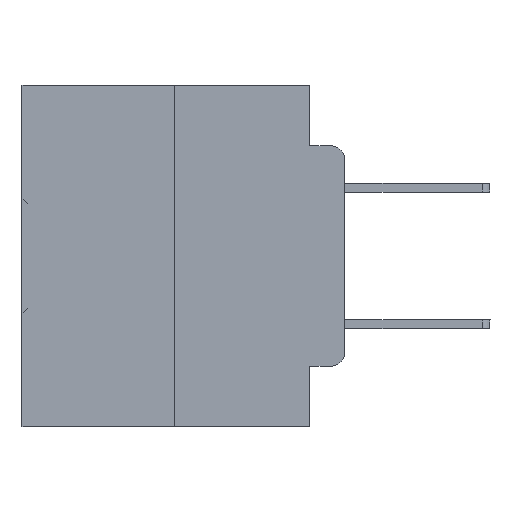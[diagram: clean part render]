
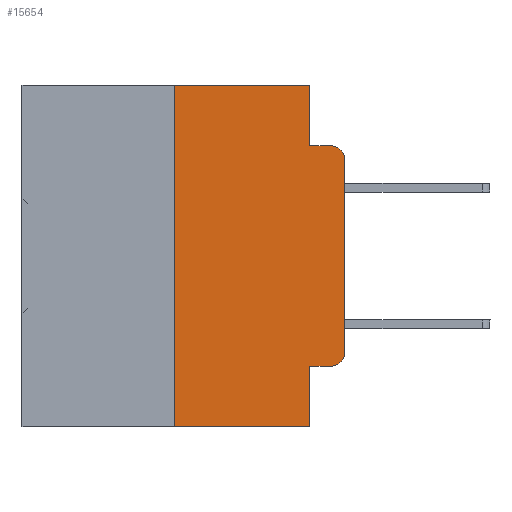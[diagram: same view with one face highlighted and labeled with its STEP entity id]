
A CAD part, left-side view. The second image highlights one B-rep face of the part: STEP entity #15654.
In plain terms, the highlighted planar face has unit normal (-1, 0, 0).
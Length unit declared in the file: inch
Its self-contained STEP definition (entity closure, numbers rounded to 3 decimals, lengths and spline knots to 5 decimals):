
#1027 = LINE ( 'NONE', #9541, #3161 ) ;
#1177 = CARTESIAN_POINT ( 'NONE',  ( 0., 0.051, 0. ) ) ;
#1514 = VERTEX_POINT ( 'NONE', #17725 ) ;
#2188 = CARTESIAN_POINT ( 'NONE',  ( 0., 0.051, -0.5 ) ) ;
#2288 = DIRECTION ( 'NONE',  ( 0., 0., -1. ) ) ;
#2424 = VECTOR ( 'NONE', #8841, 39.37008 ) ;
#2534 = CARTESIAN_POINT ( 'NONE',  ( 0., 0.051, 0. ) ) ;
#3006 = ORIENTED_EDGE ( 'NONE', *, *, #20452, .T. ) ;
#3094 = EDGE_CURVE ( 'NONE', #30216, #5274, #14071, .T. ) ;
#3161 = VECTOR ( 'NONE', #12062, 39.37008 ) ;
#3354 = CARTESIAN_POINT ( 'NONE',  ( 0., 0.25, -0.5 ) ) ;
#3765 = EDGE_CURVE ( 'NONE', #20143, #28749, #12743, .T. ) ;
#3801 = EDGE_CURVE ( 'NONE', #28749, #17695, #10401, .T. ) ;
#3813 = CARTESIAN_POINT ( 'NONE',  ( 0., 0.02, -0.4115 ) ) ;
#4164 = LINE ( 'NONE', #6699, #22034 ) ;
#4438 = DIRECTION ( 'NONE',  ( 0., 0., 1. ) ) ;
#4473 = AXIS2_PLACEMENT_3D ( 'NONE', #16022, #18914, #2288 ) ;
#4555 = VERTEX_POINT ( 'NONE', #6662 ) ;
#5274 = VERTEX_POINT ( 'NONE', #24981 ) ;
#5427 = VERTEX_POINT ( 'NONE', #3813 ) ;
#5631 = AXIS2_PLACEMENT_3D ( 'NONE', #7653, #18507, #7835 ) ;
#5682 = AXIS2_PLACEMENT_3D ( 'NONE', #30928, #16939, #17121 ) ;
#6244 = EDGE_CURVE ( 'NONE', #20143, #10310, #13314, .T. ) ;
#6662 = CARTESIAN_POINT ( 'NONE',  ( 0., 0., -0.3915 ) ) ;
#6699 = CARTESIAN_POINT ( 'NONE',  ( 0., 0.051, -0.4115 ) ) ;
#7653 = CARTESIAN_POINT ( 'NONE',  ( 0., 0.02, -0.3915 ) ) ;
#7835 = DIRECTION ( 'NONE',  ( 0., 0., -1. ) ) ;
#8578 = VECTOR ( 'NONE', #4438, 39.37008 ) ;
#8841 = DIRECTION ( 'NONE',  ( 0., -1., 0. ) ) ;
#9029 = ORIENTED_EDGE ( 'NONE', *, *, #3765, .F. ) ;
#9263 = ORIENTED_EDGE ( 'NONE', *, *, #3801, .F. ) ;
#9541 = CARTESIAN_POINT ( 'NONE',  ( 0., 0., 0. ) ) ;
#9544 = PLANE ( 'NONE',  #4473 ) ;
#10310 = VERTEX_POINT ( 'NONE', #2188 ) ;
#10401 = LINE ( 'NONE', #15629, #20732 ) ;
#10429 = EDGE_CURVE ( 'NONE', #17695, #30216, #16269, .T. ) ;
#11016 = DIRECTION ( 'NONE',  ( 0., 0., -1. ) ) ;
#11027 = EDGE_LOOP ( 'NONE', ( #29076, #34854, #33288, #33503, #9263, #9029, #14259, #21381, #15442, #3006 ) ) ;
#11551 = CARTESIAN_POINT ( 'NONE',  ( 0., 0.051, -0.0885 ) ) ;
#12062 = DIRECTION ( 'NONE',  ( 0., 0., 1. ) ) ;
#12265 = VECTOR ( 'NONE', #11016, 39.37008 ) ;
#12601 = EDGE_CURVE ( 'NONE', #4555, #27431, #1027, .T. ) ;
#12743 = LINE ( 'NONE', #26514, #8578 ) ;
#13314 = LINE ( 'NONE', #21302, #19636 ) ;
#14071 = LINE ( 'NONE', #11551, #2424 ) ;
#14259 = ORIENTED_EDGE ( 'NONE', *, *, #6244, .T. ) ;
#15009 = CARTESIAN_POINT ( 'NONE',  ( 0., 0.051, 0. ) ) ;
#15442 = ORIENTED_EDGE ( 'NONE', *, *, #30143, .T. ) ;
#15629 = CARTESIAN_POINT ( 'NONE',  ( 0., 0.473, 0. ) ) ;
#15654 = ADVANCED_FACE ( 'NONE', ( #34362 ), #9544, .F. ) ;
#16022 = CARTESIAN_POINT ( 'NONE',  ( 0., 0.473, 0. ) ) ;
#16269 = LINE ( 'NONE', #2534, #12265 ) ;
#16939 = DIRECTION ( 'NONE',  ( -1., 0., 0. ) ) ;
#17121 = DIRECTION ( 'NONE',  ( 0., 0., -1. ) ) ;
#17695 = VERTEX_POINT ( 'NONE', #15009 ) ;
#17725 = CARTESIAN_POINT ( 'NONE',  ( 0., 0.051, -0.4115 ) ) ;
#18507 = DIRECTION ( 'NONE',  ( -1., 0., 0. ) ) ;
#18718 = DIRECTION ( 'NONE',  ( 0., -1., 0. ) ) ;
#18914 = DIRECTION ( 'NONE',  ( 1., 0., 0. ) ) ;
#19356 = CARTESIAN_POINT ( 'NONE',  ( 0., 0.25, 0. ) ) ;
#19636 = VECTOR ( 'NONE', #21655, 39.37008 ) ;
#20143 = VERTEX_POINT ( 'NONE', #3354 ) ;
#20157 = CIRCLE ( 'NONE', #5682, 0.02 ) ;
#20447 = CARTESIAN_POINT ( 'NONE',  ( 0., 0.051, -0.0885 ) ) ;
#20452 = EDGE_CURVE ( 'NONE', #5427, #4555, #34583, .T. ) ;
#20732 = VECTOR ( 'NONE', #18718, 39.37008 ) ;
#21302 = CARTESIAN_POINT ( 'NONE',  ( 0., 0.473, -0.5 ) ) ;
#21381 = ORIENTED_EDGE ( 'NONE', *, *, #21713, .F. ) ;
#21576 = EDGE_CURVE ( 'NONE', #27431, #5274, #20157, .T. ) ;
#21655 = DIRECTION ( 'NONE',  ( 0., -1., 0. ) ) ;
#21713 = EDGE_CURVE ( 'NONE', #1514, #10310, #34508, .T. ) ;
#22034 = VECTOR ( 'NONE', #23704, 39.37008 ) ;
#22763 = CARTESIAN_POINT ( 'NONE',  ( 0., 0., -0.1085 ) ) ;
#23459 = DIRECTION ( 'NONE',  ( 0., 0., -1. ) ) ;
#23704 = DIRECTION ( 'NONE',  ( 0., -1., 0. ) ) ;
#24981 = CARTESIAN_POINT ( 'NONE',  ( 0., 0.02, -0.0885 ) ) ;
#26514 = CARTESIAN_POINT ( 'NONE',  ( 0., 0.25, 0. ) ) ;
#27431 = VERTEX_POINT ( 'NONE', #22763 ) ;
#28749 = VERTEX_POINT ( 'NONE', #19356 ) ;
#29076 = ORIENTED_EDGE ( 'NONE', *, *, #12601, .T. ) ;
#30143 = EDGE_CURVE ( 'NONE', #1514, #5427, #4164, .T. ) ;
#30216 = VERTEX_POINT ( 'NONE', #20447 ) ;
#30928 = CARTESIAN_POINT ( 'NONE',  ( 0., 0.02, -0.1085 ) ) ;
#33288 = ORIENTED_EDGE ( 'NONE', *, *, #3094, .F. ) ;
#33503 = ORIENTED_EDGE ( 'NONE', *, *, #10429, .F. ) ;
#34094 = VECTOR ( 'NONE', #23459, 39.37008 ) ;
#34362 = FACE_OUTER_BOUND ( 'NONE', #11027, .T. ) ;
#34508 = LINE ( 'NONE', #1177, #34094 ) ;
#34583 = CIRCLE ( 'NONE', #5631, 0.02 ) ;
#34854 = ORIENTED_EDGE ( 'NONE', *, *, #21576, .T. ) ;
